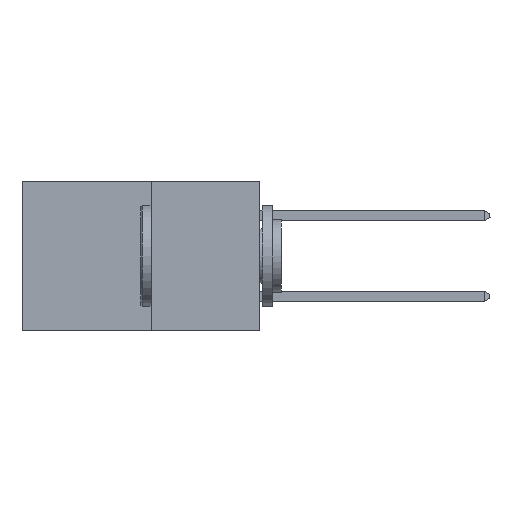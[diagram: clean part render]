
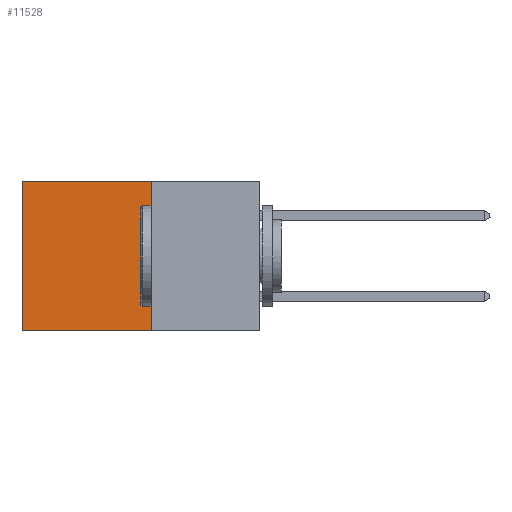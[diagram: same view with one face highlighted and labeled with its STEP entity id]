
A CAD part, left-side view. The second image highlights one B-rep face of the part: STEP entity #11528.
In plain terms, the highlighted planar face has unit normal (-1, 0, 0).
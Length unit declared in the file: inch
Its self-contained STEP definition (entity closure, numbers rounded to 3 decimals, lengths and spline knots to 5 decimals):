
#563 = LINE ( 'NONE', #18027, #5633 ) ;
#1200 = CARTESIAN_POINT ( 'NONE',  ( 0.277, 0.59, -0.37 ) ) ;
#1247 = CARTESIAN_POINT ( 'NONE',  ( 0.277, 0.27, -0.37 ) ) ;
#1727 = VECTOR ( 'NONE', #14342, 39.37008 ) ;
#2341 = LINE ( 'NONE', #16118, #18360 ) ;
#3703 = VERTEX_POINT ( 'NONE', #1200 ) ;
#3866 = VERTEX_POINT ( 'NONE', #1247 ) ;
#4602 = DIRECTION ( 'NONE',  ( 0., 1., 0. ) ) ;
#4643 = EDGE_CURVE ( 'NONE', #9434, #3866, #563, .T. ) ;
#4891 = CARTESIAN_POINT ( 'NONE',  ( 0.277, 0.27, -0.37 ) ) ;
#5174 = DIRECTION ( 'NONE',  ( 0., 0., -1. ) ) ;
#5238 = DIRECTION ( 'NONE',  ( 1., 0., 0. ) ) ;
#5541 = CARTESIAN_POINT ( 'NONE',  ( 0.277, 0.27, -0.37 ) ) ;
#5558 = PLANE ( 'NONE',  #19239 ) ;
#5633 = VECTOR ( 'NONE', #18232, 39.37008 ) ;
#6135 = LINE ( 'NONE', #4891, #14383 ) ;
#7802 = EDGE_CURVE ( 'NONE', #9434, #20911, #14469, .T. ) ;
#8344 = CARTESIAN_POINT ( 'NONE',  ( 0.277, 0.59, 0. ) ) ;
#9434 = VERTEX_POINT ( 'NONE', #17125 ) ;
#10690 = EDGE_LOOP ( 'NONE', ( #10821, #13026, #17606, #19322 ) ) ;
#10821 = ORIENTED_EDGE ( 'NONE', *, *, #16919, .T. ) ;
#11528 = ADVANCED_FACE ( 'NONE', ( #18876 ), #5558, .F. ) ;
#13026 = ORIENTED_EDGE ( 'NONE', *, *, #14314, .F. ) ;
#14314 = EDGE_CURVE ( 'NONE', #3866, #3703, #6135, .T. ) ;
#14342 = DIRECTION ( 'NONE',  ( 0., 1., 0. ) ) ;
#14383 = VECTOR ( 'NONE', #4602, 39.37008 ) ;
#14419 = CARTESIAN_POINT ( 'NONE',  ( 0.277, 0.27, 0. ) ) ;
#14469 = LINE ( 'NONE', #14419, #1727 ) ;
#16118 = CARTESIAN_POINT ( 'NONE',  ( 0.277, 0.59, -0.37 ) ) ;
#16546 = DIRECTION ( 'NONE',  ( 0., 0., -1. ) ) ;
#16919 = EDGE_CURVE ( 'NONE', #20911, #3703, #2341, .T. ) ;
#17125 = CARTESIAN_POINT ( 'NONE',  ( 0.277, 0.27, 0. ) ) ;
#17606 = ORIENTED_EDGE ( 'NONE', *, *, #4643, .F. ) ;
#18027 = CARTESIAN_POINT ( 'NONE',  ( 0.277, 0.27, -0.37 ) ) ;
#18232 = DIRECTION ( 'NONE',  ( 0., 0., -1. ) ) ;
#18360 = VECTOR ( 'NONE', #16546, 39.37008 ) ;
#18876 = FACE_OUTER_BOUND ( 'NONE', #10690, .T. ) ;
#19239 = AXIS2_PLACEMENT_3D ( 'NONE', #5541, #5238, #5174 ) ;
#19322 = ORIENTED_EDGE ( 'NONE', *, *, #7802, .T. ) ;
#20911 = VERTEX_POINT ( 'NONE', #8344 ) ;
